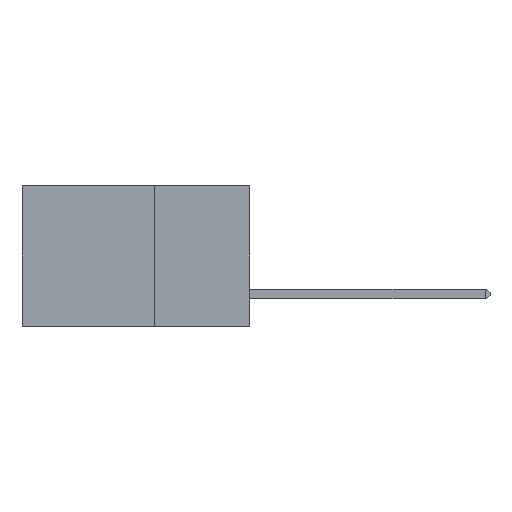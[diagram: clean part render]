
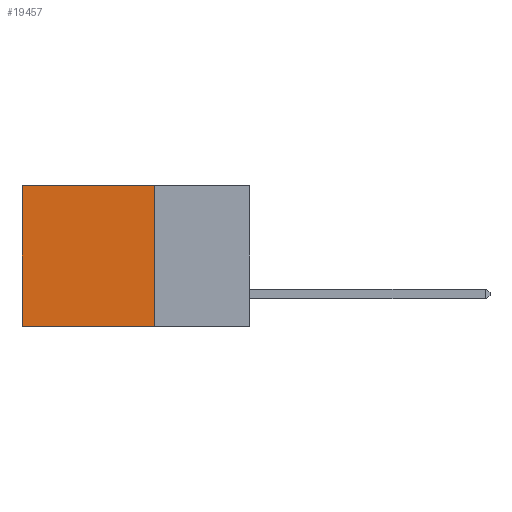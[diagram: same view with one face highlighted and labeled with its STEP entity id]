
A CAD part, left-side view. The second image highlights one B-rep face of the part: STEP entity #19457.
In plain terms, the highlighted planar face has unit normal (-1, 0, 0).
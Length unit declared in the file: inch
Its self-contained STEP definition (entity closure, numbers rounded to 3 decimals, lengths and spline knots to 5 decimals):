
#259 = ORIENTED_EDGE ( 'NONE', *, *, #20145, .T. ) ;
#1177 = CARTESIAN_POINT ( 'NONE',  ( 0.2875, 0.6, 0. ) ) ;
#1552 = FACE_OUTER_BOUND ( 'NONE', #12406, .T. ) ;
#1905 = CARTESIAN_POINT ( 'NONE',  ( 0.2875, 0.25, 0. ) ) ;
#1986 = DIRECTION ( 'NONE',  ( 0., 1., 0. ) ) ;
#3122 = LINE ( 'NONE', #19739, #9088 ) ;
#3414 = LINE ( 'NONE', #5560, #13764 ) ;
#3615 = DIRECTION ( 'NONE',  ( 0., 0., -1. ) ) ;
#4200 = CARTESIAN_POINT ( 'NONE',  ( 0.2875, 0.25, -0.37 ) ) ;
#4476 = DIRECTION ( 'NONE',  ( 0., 0., -1. ) ) ;
#5225 = CARTESIAN_POINT ( 'NONE',  ( 0.2875, 0.6, -0.37 ) ) ;
#5560 = CARTESIAN_POINT ( 'NONE',  ( 0.2875, 0.25, -0.37 ) ) ;
#5944 = VERTEX_POINT ( 'NONE', #14359 ) ;
#6207 = VERTEX_POINT ( 'NONE', #5225 ) ;
#7772 = AXIS2_PLACEMENT_3D ( 'NONE', #31448, #18827, #3615 ) ;
#8971 = EDGE_CURVE ( 'NONE', #5944, #14853, #3122, .T. ) ;
#9088 = VECTOR ( 'NONE', #1986, 39.37008 ) ;
#10188 = ORIENTED_EDGE ( 'NONE', *, *, #8971, .T. ) ;
#10554 = EDGE_CURVE ( 'NONE', #22792, #6207, #3414, .T. ) ;
#11040 = ORIENTED_EDGE ( 'NONE', *, *, #10554, .F. ) ;
#12406 = EDGE_LOOP ( 'NONE', ( #259, #11040, #12480, #10188 ) ) ;
#12480 = ORIENTED_EDGE ( 'NONE', *, *, #22633, .F. ) ;
#13764 = VECTOR ( 'NONE', #20754, 39.37008 ) ;
#14359 = CARTESIAN_POINT ( 'NONE',  ( 0.2875, 0.25, 0. ) ) ;
#14846 = LINE ( 'NONE', #1905, #27547 ) ;
#14853 = VERTEX_POINT ( 'NONE', #1177 ) ;
#17789 = VECTOR ( 'NONE', #32201, 39.37008 ) ;
#18827 = DIRECTION ( 'NONE',  ( 1., 0., 0. ) ) ;
#19457 = ADVANCED_FACE ( 'NONE', ( #1552 ), #28926, .F. ) ;
#19739 = CARTESIAN_POINT ( 'NONE',  ( 0.2875, 0.25, 0. ) ) ;
#20145 = EDGE_CURVE ( 'NONE', #14853, #6207, #24543, .T. ) ;
#20754 = DIRECTION ( 'NONE',  ( 0., 1., 0. ) ) ;
#22024 = CARTESIAN_POINT ( 'NONE',  ( 0.2875, 0.6, 0. ) ) ;
#22633 = EDGE_CURVE ( 'NONE', #5944, #22792, #14846, .T. ) ;
#22792 = VERTEX_POINT ( 'NONE', #4200 ) ;
#24543 = LINE ( 'NONE', #22024, #17789 ) ;
#27547 = VECTOR ( 'NONE', #4476, 39.37008 ) ;
#28926 = PLANE ( 'NONE',  #7772 ) ;
#31448 = CARTESIAN_POINT ( 'NONE',  ( 0.2875, 0.25, 0. ) ) ;
#32201 = DIRECTION ( 'NONE',  ( 0., 0., -1. ) ) ;
